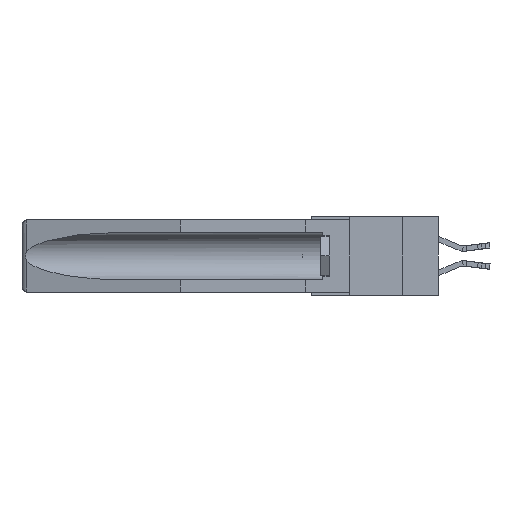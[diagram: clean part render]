
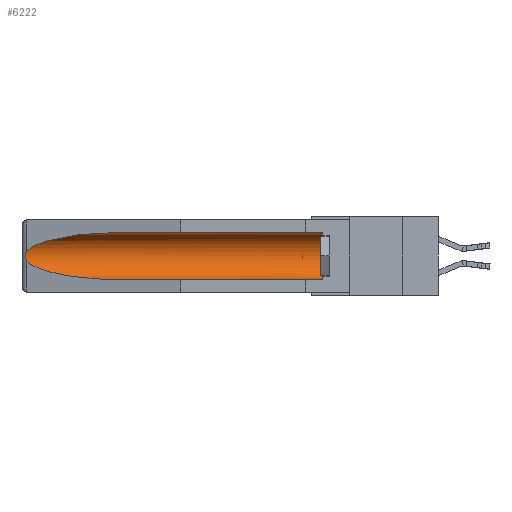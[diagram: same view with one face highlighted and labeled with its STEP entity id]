
A CAD part, left-side view. The second image highlights one B-rep face of the part: STEP entity #6222.
In plain terms, the highlighted cylindrical face has radius 2.857 mm (diameter 5.715 mm), a partial arc.
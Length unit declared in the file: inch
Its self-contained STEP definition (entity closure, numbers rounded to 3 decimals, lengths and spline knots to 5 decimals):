
#124 = CARTESIAN_POINT ( 'NONE',  ( 0.155, 1.07973, -0.059 ) ) ;
#442 = CARTESIAN_POINT ( 'NONE',  ( 0.26655, 1.53094, -0.18657 ) ) ;
#1174 = CARTESIAN_POINT ( 'NONE',  ( 0.155, -0.30754, -0.284 ) ) ;
#1627 = DIRECTION ( 'NONE',  ( 0., 0., 1. ) ) ;
#2153 = EDGE_CURVE ( 'NONE', #4767, #23233, #10934, .T. ) ;
#3009 = CARTESIAN_POINT ( 'NONE',  ( 0.26537, 1.52718, -0.19328 ) ) ;
#3087 = CARTESIAN_POINT ( 'NONE',  ( 0.21114, 1.30732, -0.059 ) ) ;
#4345 = EDGE_CURVE ( 'NONE', #23233, #32905, #11839, .T. ) ;
#4365 = CARTESIAN_POINT ( 'NONE',  ( 0.25451, 1.48313, -0.24835 ) ) ;
#4669 = DIRECTION ( 'NONE',  ( 0., 1., 0. ) ) ;
#4767 = VERTEX_POINT ( 'NONE', #23293 ) ;
#5598 = ORIENTED_EDGE ( 'NONE', *, *, #4345, .T. ) ;
#6222 = ADVANCED_FACE ( 'NONE', ( #23241 ), #7485, .F. ) ;
#6454 = DIRECTION ( 'NONE',  ( 0., 0., 1. ) ) ;
#7485 = CYLINDRICAL_SURFACE ( 'NONE', #8053, 0.1125 ) ;
#7852 = EDGE_CURVE ( 'NONE', #13416, #32905, #35308, .T. ) ;
#8053 = AXIS2_PLACEMENT_3D ( 'NONE', #29816, #4669, #1627 ) ;
#8332 = CARTESIAN_POINT ( 'NONE',  ( 0.155, -0.30754, -0.059 ) ) ;
#8451 = DIRECTION ( 'NONE',  ( 0., 1., 0. ) ) ;
#8579 = CARTESIAN_POINT ( 'NONE',  ( 0.26537, 1.52718, -0.14972 ) ) ;
#8748 = VECTOR ( 'NONE', #8451, 39.37008 ) ;
#8864 = CARTESIAN_POINT ( 'NONE',  ( 0.26597, 1.5296, -0.19026 ) ) ;
#9489 = CARTESIAN_POINT ( 'NONE',  ( 0.155, 1.07973, -0.284 ) ) ;
#10934 = B_SPLINE_CURVE_WITH_KNOTS ( 'NONE', 3,
 ( #14255, #17185, #33990, #22896, #33762, #19636, #25213, #442, #8864, #3009 ),
 .UNSPECIFIED., .F., .F.,
 ( 4, 2, 2, 2, 4 ),
 ( 0., 0.00029, 0.00058, 0.00087, 0.00117 ),
 .UNSPECIFIED. ) ;
#11839 =( BOUNDED_CURVE ( )  B_SPLINE_CURVE ( 3, ( #26355, #4365, #23425, #9489 ),
 .UNSPECIFIED., .F., .F. ) 
 B_SPLINE_CURVE_WITH_KNOTS ( ( 4, 4 ),
 ( 0.1948, 1.5708 ),
 .UNSPECIFIED. ) 
 CURVE ( )  GEOMETRIC_REPRESENTATION_ITEM ( )  RATIONAL_B_SPLINE_CURVE ( ( 1., 0.848, 0.848, 1. ) ) 
 REPRESENTATION_ITEM ( '' )  );
#11848 = ORIENTED_EDGE ( 'NONE', *, *, #2153, .T. ) ;
#13135 = AXIS2_PLACEMENT_3D ( 'NONE', #20501, #15021, #6454 ) ;
#13416 = VERTEX_POINT ( 'NONE', #23663 ) ;
#13808 = ORIENTED_EDGE ( 'NONE', *, *, #24205, .T. ) ;
#14255 = CARTESIAN_POINT ( 'NONE',  ( 0.26537, 1.52718, -0.14972 ) ) ;
#15021 = DIRECTION ( 'NONE',  ( 0., -1., 0. ) ) ;
#16758 = CIRCLE ( 'NONE', #13135, 0.1125 ) ;
#16794 = CARTESIAN_POINT ( 'NONE',  ( 0.26537, 1.52718, -0.19328 ) ) ;
#17185 = CARTESIAN_POINT ( 'NONE',  ( 0.26597, 1.52961, -0.15275 ) ) ;
#18067 = EDGE_CURVE ( 'NONE', #23318, #32782, #18819, .T. ) ;
#18819 = LINE ( 'NONE', #8332, #8748 ) ;
#19636 = CARTESIAN_POINT ( 'NONE',  ( 0.2675, 1.53308, -0.17534 ) ) ;
#19689 =( BOUNDED_CURVE ( )  B_SPLINE_CURVE ( 3, ( #25286, #3087, #22853, #8579 ),
 .UNSPECIFIED., .F., .F. ) 
 B_SPLINE_CURVE_WITH_KNOTS ( ( 4, 4 ),
 ( 4.71239, 6.08839 ),
 .UNSPECIFIED. ) 
 CURVE ( )  GEOMETRIC_REPRESENTATION_ITEM ( )  RATIONAL_B_SPLINE_CURVE ( ( 1., 0.848, 0.848, 1. ) ) 
 REPRESENTATION_ITEM ( '' )  );
#20501 = CARTESIAN_POINT ( 'NONE',  ( 0.155, 0.126, -0.1715 ) ) ;
#22473 = EDGE_LOOP ( 'NONE', ( #13808, #11848, #5598, #33641, #33387, #34741 ) ) ;
#22853 = CARTESIAN_POINT ( 'NONE',  ( 0.25451, 1.48313, -0.09465 ) ) ;
#22896 = CARTESIAN_POINT ( 'NONE',  ( 0.2673, 1.5327, -0.16383 ) ) ;
#23185 = CARTESIAN_POINT ( 'NONE',  ( 0.155, 1.07973, -0.284 ) ) ;
#23233 = VERTEX_POINT ( 'NONE', #16794 ) ;
#23241 = FACE_OUTER_BOUND ( 'NONE', #22473, .T. ) ;
#23293 = CARTESIAN_POINT ( 'NONE',  ( 0.26537, 1.52718, -0.14972 ) ) ;
#23318 = VERTEX_POINT ( 'NONE', #34195 ) ;
#23425 = CARTESIAN_POINT ( 'NONE',  ( 0.21114, 1.30732, -0.284 ) ) ;
#23663 = CARTESIAN_POINT ( 'NONE',  ( 0.155, 0.126, -0.284 ) ) ;
#23879 = DIRECTION ( 'NONE',  ( 0., 1., 0. ) ) ;
#24205 = EDGE_CURVE ( 'NONE', #32782, #4767, #19689, .T. ) ;
#25213 = CARTESIAN_POINT ( 'NONE',  ( 0.2673, 1.53269, -0.17917 ) ) ;
#25286 = CARTESIAN_POINT ( 'NONE',  ( 0.155, 1.07973, -0.059 ) ) ;
#26355 = CARTESIAN_POINT ( 'NONE',  ( 0.26537, 1.52718, -0.19328 ) ) ;
#29633 = VECTOR ( 'NONE', #23879, 39.37008 ) ;
#29816 = CARTESIAN_POINT ( 'NONE',  ( 0.155, -0.30754, -0.1715 ) ) ;
#32782 = VERTEX_POINT ( 'NONE', #124 ) ;
#32905 = VERTEX_POINT ( 'NONE', #23185 ) ;
#33387 = ORIENTED_EDGE ( 'NONE', *, *, #35995, .T. ) ;
#33641 = ORIENTED_EDGE ( 'NONE', *, *, #7852, .F. ) ;
#33762 = CARTESIAN_POINT ( 'NONE',  ( 0.2675, 1.53308, -0.16763 ) ) ;
#33990 = CARTESIAN_POINT ( 'NONE',  ( 0.26654, 1.53092, -0.15636 ) ) ;
#34195 = CARTESIAN_POINT ( 'NONE',  ( 0.155, 0.126, -0.059 ) ) ;
#34741 = ORIENTED_EDGE ( 'NONE', *, *, #18067, .T. ) ;
#35308 = LINE ( 'NONE', #1174, #29633 ) ;
#35995 = EDGE_CURVE ( 'NONE', #13416, #23318, #16758, .T. ) ;
